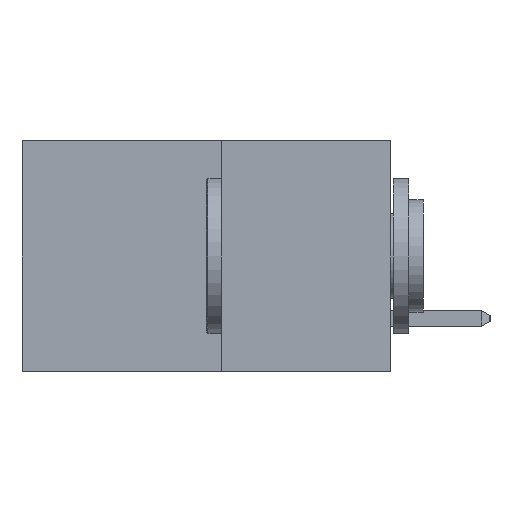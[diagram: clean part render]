
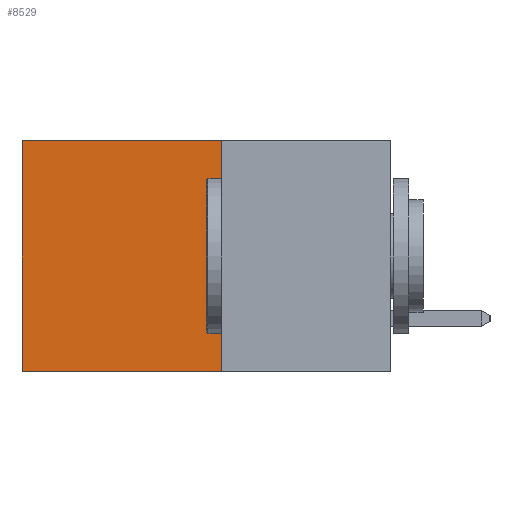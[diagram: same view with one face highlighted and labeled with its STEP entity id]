
A CAD part, left-side view. The second image highlights one B-rep face of the part: STEP entity #8529.
In plain terms, the highlighted planar face has unit normal (-1, 0, 0).
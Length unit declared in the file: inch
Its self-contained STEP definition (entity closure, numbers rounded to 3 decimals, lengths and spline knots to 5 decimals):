
#19 = AXIS2_PLACEMENT_3D ( 'NONE', #6816, #6903, #6675 ) ;
#393 = CARTESIAN_POINT ( 'NONE',  ( 0.277, 0.27, -0.37 ) ) ;
#509 = CARTESIAN_POINT ( 'NONE',  ( 0.277, 0.59, 0. ) ) ;
#2017 = VECTOR ( 'NONE', #9344, 39.37008 ) ;
#2180 = EDGE_CURVE ( 'NONE', #10669, #2369, #7345, .T. ) ;
#2369 = VERTEX_POINT ( 'NONE', #393 ) ;
#2416 = ORIENTED_EDGE ( 'NONE', *, *, #12607, .T. ) ;
#2804 = EDGE_LOOP ( 'NONE', ( #2416, #10220, #8356, #8555 ) ) ;
#4286 = DIRECTION ( 'NONE',  ( 0., 1., 0. ) ) ;
#4471 = CARTESIAN_POINT ( 'NONE',  ( 0.277, 0.27, 0. ) ) ;
#4510 = CARTESIAN_POINT ( 'NONE',  ( 0.277, 0.27, -0.37 ) ) ;
#4570 = VERTEX_POINT ( 'NONE', #6995 ) ;
#4692 = DIRECTION ( 'NONE',  ( 0., 0., -1. ) ) ;
#4791 = EDGE_CURVE ( 'NONE', #10669, #5093, #7437, .T. ) ;
#5093 = VERTEX_POINT ( 'NONE', #509 ) ;
#6498 = DIRECTION ( 'NONE',  ( 0., 1., 0. ) ) ;
#6675 = DIRECTION ( 'NONE',  ( 0., 0., -1. ) ) ;
#6694 = PLANE ( 'NONE',  #19 ) ;
#6816 = CARTESIAN_POINT ( 'NONE',  ( 0.277, 0.27, -0.37 ) ) ;
#6903 = DIRECTION ( 'NONE',  ( 1., 0., 0. ) ) ;
#6995 = CARTESIAN_POINT ( 'NONE',  ( 0.277, 0.59, -0.37 ) ) ;
#7345 = LINE ( 'NONE', #4510, #10405 ) ;
#7373 = LINE ( 'NONE', #8442, #2017 ) ;
#7437 = LINE ( 'NONE', #4471, #12091 ) ;
#8356 = ORIENTED_EDGE ( 'NONE', *, *, #2180, .F. ) ;
#8442 = CARTESIAN_POINT ( 'NONE',  ( 0.277, 0.59, -0.37 ) ) ;
#8529 = ADVANCED_FACE ( 'NONE', ( #11978 ), #6694, .F. ) ;
#8555 = ORIENTED_EDGE ( 'NONE', *, *, #4791, .T. ) ;
#9307 = VECTOR ( 'NONE', #6498, 39.37008 ) ;
#9344 = DIRECTION ( 'NONE',  ( 0., 0., -1. ) ) ;
#9593 = LINE ( 'NONE', #10222, #9307 ) ;
#10220 = ORIENTED_EDGE ( 'NONE', *, *, #10404, .F. ) ;
#10222 = CARTESIAN_POINT ( 'NONE',  ( 0.277, 0.27, -0.37 ) ) ;
#10404 = EDGE_CURVE ( 'NONE', #2369, #4570, #9593, .T. ) ;
#10405 = VECTOR ( 'NONE', #4692, 39.37008 ) ;
#10669 = VERTEX_POINT ( 'NONE', #12498 ) ;
#11978 = FACE_OUTER_BOUND ( 'NONE', #2804, .T. ) ;
#12091 = VECTOR ( 'NONE', #4286, 39.37008 ) ;
#12498 = CARTESIAN_POINT ( 'NONE',  ( 0.277, 0.27, 0. ) ) ;
#12607 = EDGE_CURVE ( 'NONE', #5093, #4570, #7373, .T. ) ;
